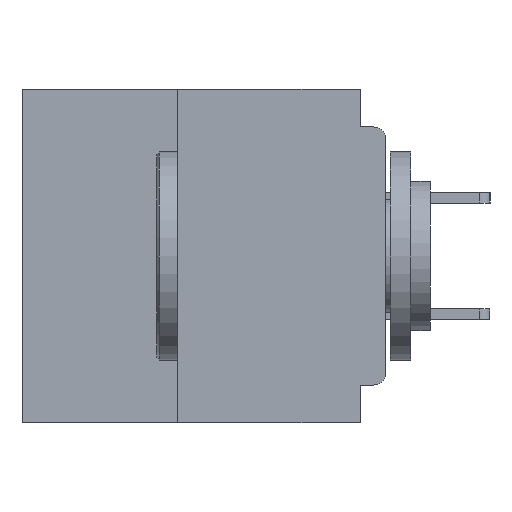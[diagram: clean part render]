
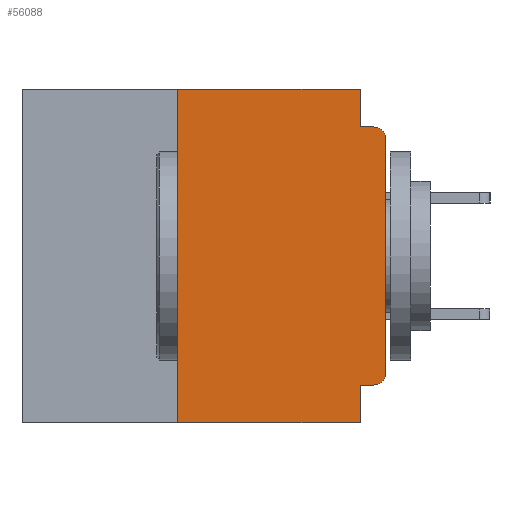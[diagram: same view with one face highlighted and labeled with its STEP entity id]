
A CAD part, left-side view. The second image highlights one B-rep face of the part: STEP entity #56088.
In plain terms, the highlighted planar face has unit normal (-1, 0, 0).
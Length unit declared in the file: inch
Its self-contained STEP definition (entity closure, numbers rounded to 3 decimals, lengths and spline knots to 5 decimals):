
#109 = CARTESIAN_POINT ( 'NONE',  ( 0., 0.25, -0.4 ) ) ;
#2531 = EDGE_CURVE ( 'NONE', #59907, #32507, #45747, .T. ) ;
#3743 = ORIENTED_EDGE ( 'NONE', *, *, #32540, .F. ) ;
#5083 = EDGE_CURVE ( 'NONE', #44064, #26294, #13930, .T. ) ;
#5539 = CARTESIAN_POINT ( 'NONE',  ( 0., 0.031, -0.4 ) ) ;
#5749 = LINE ( 'NONE', #15386, #53993 ) ;
#5823 = CARTESIAN_POINT ( 'NONE',  ( 0., 0.015, -0.045 ) ) ;
#6033 = CARTESIAN_POINT ( 'NONE',  ( 0., 0.031, 0. ) ) ;
#6550 = ORIENTED_EDGE ( 'NONE', *, *, #5083, .F. ) ;
#8439 = CARTESIAN_POINT ( 'NONE',  ( 0., 0., -0.34 ) ) ;
#9076 = ORIENTED_EDGE ( 'NONE', *, *, #32616, .T. ) ;
#11052 = DIRECTION ( 'NONE',  ( -1., 0., 0. ) ) ;
#11232 = DIRECTION ( 'NONE',  ( 0., 0., 1. ) ) ;
#12011 = VECTOR ( 'NONE', #53695, 39.37008 ) ;
#12251 = AXIS2_PLACEMENT_3D ( 'NONE', #35974, #45351, #17335 ) ;
#12603 = PLANE ( 'NONE',  #12251 ) ;
#12902 = ORIENTED_EDGE ( 'NONE', *, *, #29121, .F. ) ;
#13783 = AXIS2_PLACEMENT_3D ( 'NONE', #31804, #31796, #31748 ) ;
#13930 = LINE ( 'NONE', #29562, #49751 ) ;
#15386 = CARTESIAN_POINT ( 'NONE',  ( 0., 0., -0.045 ) ) ;
#17113 = EDGE_CURVE ( 'NONE', #54332, #44064, #52392, .T. ) ;
#17335 = DIRECTION ( 'NONE',  ( 0., 0., -1. ) ) ;
#18326 = VERTEX_POINT ( 'NONE', #109 ) ;
#19832 = CARTESIAN_POINT ( 'NONE',  ( 0., 0.25, 0. ) ) ;
#20545 = ORIENTED_EDGE ( 'NONE', *, *, #59757, .F. ) ;
#21097 = CARTESIAN_POINT ( 'NONE',  ( 0., 0., -0.355 ) ) ;
#22675 = VECTOR ( 'NONE', #11232, 39.37008 ) ;
#24131 = LINE ( 'NONE', #53122, #22675 ) ;
#24338 = LINE ( 'NONE', #25797, #47733 ) ;
#24720 = DIRECTION ( 'NONE',  ( 0., 0., 1. ) ) ;
#25118 = VECTOR ( 'NONE', #24720, 39.37008 ) ;
#25371 = VERTEX_POINT ( 'NONE', #8439 ) ;
#25797 = CARTESIAN_POINT ( 'NONE',  ( 0., 0.437, -0.4 ) ) ;
#26093 = ORIENTED_EDGE ( 'NONE', *, *, #39082, .T. ) ;
#26294 = VERTEX_POINT ( 'NONE', #48250 ) ;
#26415 = VERTEX_POINT ( 'NONE', #39689 ) ;
#26861 = VERTEX_POINT ( 'NONE', #54949 ) ;
#27847 = EDGE_CURVE ( 'NONE', #25371, #59907, #49921, .T. ) ;
#28942 = DIRECTION ( 'NONE',  ( 0., 0., -1. ) ) ;
#29121 = EDGE_CURVE ( 'NONE', #18326, #54332, #24131, .T. ) ;
#29562 = CARTESIAN_POINT ( 'NONE',  ( 0., 0.031, 0. ) ) ;
#30536 = DIRECTION ( 'NONE',  ( 0., -1., 0. ) ) ;
#31748 = DIRECTION ( 'NONE',  ( 0., 0., -1. ) ) ;
#31796 = DIRECTION ( 'NONE',  ( -1., 0., 0. ) ) ;
#31804 = CARTESIAN_POINT ( 'NONE',  ( 0., 0.015, -0.06 ) ) ;
#32507 = VERTEX_POINT ( 'NONE', #5823 ) ;
#32540 = EDGE_CURVE ( 'NONE', #26415, #34273, #42726, .T. ) ;
#32616 = EDGE_CURVE ( 'NONE', #26861, #25371, #39788, .T. ) ;
#34045 = ORIENTED_EDGE ( 'NONE', *, *, #17113, .F. ) ;
#34273 = VERTEX_POINT ( 'NONE', #37554 ) ;
#35974 = CARTESIAN_POINT ( 'NONE',  ( 0., 0.437, 0. ) ) ;
#36022 = CARTESIAN_POINT ( 'NONE',  ( 0., 0., -0.06 ) ) ;
#36967 = LINE ( 'NONE', #21097, #12011 ) ;
#37117 = VECTOR ( 'NONE', #41846, 39.37008 ) ;
#37149 = CARTESIAN_POINT ( 'NONE',  ( 0., 0.437, 0. ) ) ;
#37554 = CARTESIAN_POINT ( 'NONE',  ( 0., 0.031, -0.4 ) ) ;
#39082 = EDGE_CURVE ( 'NONE', #18326, #34273, #24338, .T. ) ;
#39149 = CARTESIAN_POINT ( 'NONE',  ( 0., 0.015, -0.34 ) ) ;
#39689 = CARTESIAN_POINT ( 'NONE',  ( 0., 0.031, -0.355 ) ) ;
#39788 = CIRCLE ( 'NONE', #44988, 0.015 ) ;
#41846 = DIRECTION ( 'NONE',  ( 0., -1., 0. ) ) ;
#42726 = LINE ( 'NONE', #5539, #55003 ) ;
#43434 = DIRECTION ( 'NONE',  ( 0., -1., 0. ) ) ;
#43449 = DIRECTION ( 'NONE',  ( 0., 0., -1. ) ) ;
#43839 = DIRECTION ( 'NONE',  ( 0., 0., -1. ) ) ;
#44064 = VERTEX_POINT ( 'NONE', #6033 ) ;
#44988 = AXIS2_PLACEMENT_3D ( 'NONE', #39149, #11052, #43839 ) ;
#45351 = DIRECTION ( 'NONE',  ( 1., 0., 0. ) ) ;
#45747 = CIRCLE ( 'NONE', #13783, 0.015 ) ;
#46256 = ORIENTED_EDGE ( 'NONE', *, *, #2531, .T. ) ;
#47733 = VECTOR ( 'NONE', #30536, 39.37008 ) ;
#47949 = EDGE_CURVE ( 'NONE', #26294, #32507, #5749, .T. ) ;
#48250 = CARTESIAN_POINT ( 'NONE',  ( 0., 0.031, -0.045 ) ) ;
#49751 = VECTOR ( 'NONE', #43449, 39.37008 ) ;
#49921 = LINE ( 'NONE', #52644, #25118 ) ;
#51192 = FACE_OUTER_BOUND ( 'NONE', #54764, .T. ) ;
#52392 = LINE ( 'NONE', #37149, #37117 ) ;
#52633 = ORIENTED_EDGE ( 'NONE', *, *, #47949, .F. ) ;
#52644 = CARTESIAN_POINT ( 'NONE',  ( 0., 0., 0. ) ) ;
#53122 = CARTESIAN_POINT ( 'NONE',  ( 0., 0.25, -0.4 ) ) ;
#53695 = DIRECTION ( 'NONE',  ( 0., 1., 0. ) ) ;
#53993 = VECTOR ( 'NONE', #43434, 39.37008 ) ;
#54332 = VERTEX_POINT ( 'NONE', #19832 ) ;
#54764 = EDGE_LOOP ( 'NONE', ( #57349, #46256, #52633, #6550, #34045, #12902, #26093, #3743, #20545, #9076 ) ) ;
#54949 = CARTESIAN_POINT ( 'NONE',  ( 0., 0.015, -0.355 ) ) ;
#55003 = VECTOR ( 'NONE', #28942, 39.37008 ) ;
#56088 = ADVANCED_FACE ( 'NONE', ( #51192 ), #12603, .F. ) ;
#57349 = ORIENTED_EDGE ( 'NONE', *, *, #27847, .T. ) ;
#59757 = EDGE_CURVE ( 'NONE', #26861, #26415, #36967, .T. ) ;
#59907 = VERTEX_POINT ( 'NONE', #36022 ) ;
